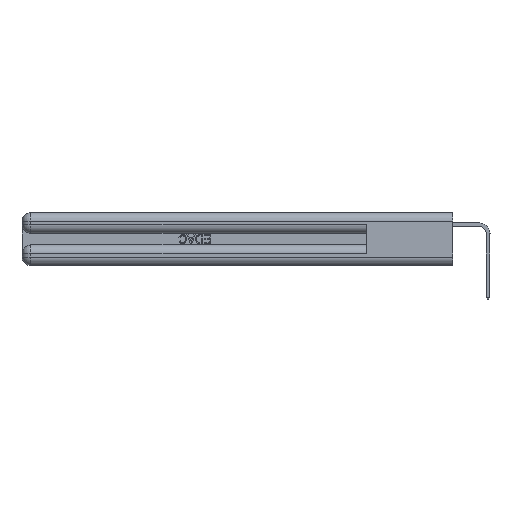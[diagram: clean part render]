
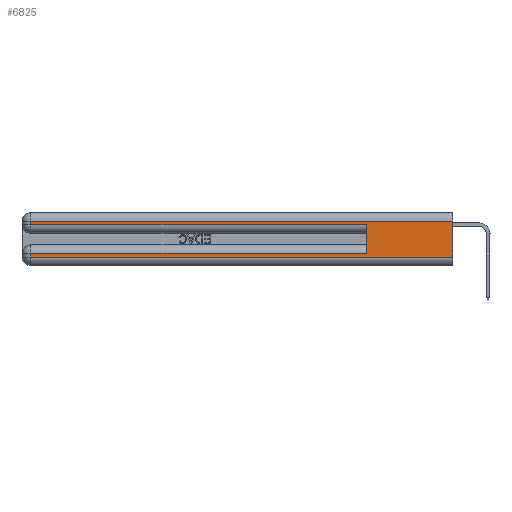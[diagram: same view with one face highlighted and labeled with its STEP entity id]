
A CAD part, left-side view. The second image highlights one B-rep face of the part: STEP entity #6825.
In plain terms, the highlighted planar face has unit normal (-1, 0, 0).
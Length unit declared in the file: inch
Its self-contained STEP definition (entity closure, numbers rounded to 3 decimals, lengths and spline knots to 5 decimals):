
#424 = VERTEX_POINT ( 'NONE', #33444 ) ;
#1484 = CARTESIAN_POINT ( 'NONE',  ( 0., 0., 0.06 ) ) ;
#2263 = DIRECTION ( 'NONE',  ( 0., -1., 0. ) ) ;
#2426 = CARTESIAN_POINT ( 'NONE',  ( 0., 0., 0.31 ) ) ;
#2656 = DIRECTION ( 'NONE',  ( 0., 0., -1. ) ) ;
#2927 = CARTESIAN_POINT ( 'NONE',  ( 0., 0., 0.06 ) ) ;
#2963 = EDGE_CURVE ( 'NONE', #10568, #35338, #14637, .T. ) ;
#3286 = CARTESIAN_POINT ( 'NONE',  ( 0., 0., 0.085 ) ) ;
#4837 = ORIENTED_EDGE ( 'NONE', *, *, #39243, .F. ) ;
#4884 = ORIENTED_EDGE ( 'NONE', *, *, #37162, .T. ) ;
#5134 = EDGE_CURVE ( 'NONE', #16854, #10568, #35204, .T. ) ;
#5466 = ORIENTED_EDGE ( 'NONE', *, *, #28726, .T. ) ;
#5582 = CARTESIAN_POINT ( 'NONE',  ( 0., 2.94, 0.37 ) ) ;
#6141 = FACE_OUTER_BOUND ( 'NONE', #28118, .T. ) ;
#6329 = ORIENTED_EDGE ( 'NONE', *, *, #24463, .T. ) ;
#6825 = ADVANCED_FACE ( 'NONE', ( #6141 ), #37628, .F. ) ;
#6867 = ORIENTED_EDGE ( 'NONE', *, *, #13900, .F. ) ;
#6901 = ORIENTED_EDGE ( 'NONE', *, *, #11723, .T. ) ;
#6944 = VERTEX_POINT ( 'NONE', #25772 ) ;
#7270 = LINE ( 'NONE', #40401, #31692 ) ;
#7369 = ORIENTED_EDGE ( 'NONE', *, *, #5134, .T. ) ;
#7371 = VECTOR ( 'NONE', #28893, 39.37008 ) ;
#7426 = DIRECTION ( 'NONE',  ( 0., 0., -1. ) ) ;
#8415 = ORIENTED_EDGE ( 'NONE', *, *, #2963, .T. ) ;
#9914 = VECTOR ( 'NONE', #27949, 39.37008 ) ;
#10568 = VERTEX_POINT ( 'NONE', #36008 ) ;
#11723 = EDGE_CURVE ( 'NONE', #34550, #16854, #15983, .T. ) ;
#11969 = CARTESIAN_POINT ( 'NONE',  ( 0., 0.6, 0.085 ) ) ;
#13226 = CARTESIAN_POINT ( 'NONE',  ( 0., 0.6, 0.145 ) ) ;
#13900 = EDGE_CURVE ( 'NONE', #34550, #424, #19579, .T. ) ;
#14637 = LINE ( 'NONE', #1484, #30477 ) ;
#15983 = LINE ( 'NONE', #3286, #7371 ) ;
#16854 = VERTEX_POINT ( 'NONE', #33305 ) ;
#17911 = CARTESIAN_POINT ( 'NONE',  ( 0., 2.94, 0.37 ) ) ;
#18240 = LINE ( 'NONE', #2426, #20194 ) ;
#18778 = CARTESIAN_POINT ( 'NONE',  ( 0., 0., 0.37 ) ) ;
#18879 = VECTOR ( 'NONE', #33598, 39.37008 ) ;
#19579 = LINE ( 'NONE', #13226, #37330 ) ;
#20194 = VECTOR ( 'NONE', #24873, 39.37008 ) ;
#21953 = DIRECTION ( 'NONE',  ( 1., 0., 0. ) ) ;
#22885 = VECTOR ( 'NONE', #7426, 39.37008 ) ;
#23954 = DIRECTION ( 'NONE',  ( 0., -1., 0. ) ) ;
#24463 = EDGE_CURVE ( 'NONE', #28976, #424, #7270, .T. ) ;
#24873 = DIRECTION ( 'NONE',  ( 0., 1., 0. ) ) ;
#25772 = CARTESIAN_POINT ( 'NONE',  ( 0., 2.94, 0.31 ) ) ;
#25849 = LINE ( 'NONE', #29750, #22885 ) ;
#27949 = DIRECTION ( 'NONE',  ( 0., 0., -1. ) ) ;
#28118 = EDGE_LOOP ( 'NONE', ( #4837, #4884, #5466, #6329, #6867, #6901, #7369, #8415 ) ) ;
#28726 = EDGE_CURVE ( 'NONE', #6944, #28976, #29244, .T. ) ;
#28893 = DIRECTION ( 'NONE',  ( 0., 1., 0. ) ) ;
#28976 = VERTEX_POINT ( 'NONE', #41105 ) ;
#29191 = VERTEX_POINT ( 'NONE', #35911 ) ;
#29244 = LINE ( 'NONE', #17911, #18879 ) ;
#29750 = CARTESIAN_POINT ( 'NONE',  ( 0., 0., 0.37 ) ) ;
#30477 = VECTOR ( 'NONE', #23954, 39.37008 ) ;
#31692 = VECTOR ( 'NONE', #2263, 39.37008 ) ;
#32204 = AXIS2_PLACEMENT_3D ( 'NONE', #18778, #21953, #2656 ) ;
#33305 = CARTESIAN_POINT ( 'NONE',  ( 0., 2.94, 0.085 ) ) ;
#33444 = CARTESIAN_POINT ( 'NONE',  ( 0., 0.6, 0.285 ) ) ;
#33598 = DIRECTION ( 'NONE',  ( 0., 0., -1. ) ) ;
#34550 = VERTEX_POINT ( 'NONE', #11969 ) ;
#35204 = LINE ( 'NONE', #5582, #9914 ) ;
#35318 = DIRECTION ( 'NONE',  ( 0., 0., 1. ) ) ;
#35338 = VERTEX_POINT ( 'NONE', #2927 ) ;
#35911 = CARTESIAN_POINT ( 'NONE',  ( 0., 0., 0.31 ) ) ;
#36008 = CARTESIAN_POINT ( 'NONE',  ( 0., 2.94, 0.06 ) ) ;
#37162 = EDGE_CURVE ( 'NONE', #29191, #6944, #18240, .T. ) ;
#37330 = VECTOR ( 'NONE', #35318, 39.37008 ) ;
#37628 = PLANE ( 'NONE',  #32204 ) ;
#39243 = EDGE_CURVE ( 'NONE', #29191, #35338, #25849, .T. ) ;
#40401 = CARTESIAN_POINT ( 'NONE',  ( 0., 0., 0.285 ) ) ;
#41105 = CARTESIAN_POINT ( 'NONE',  ( 0., 2.94, 0.285 ) ) ;
